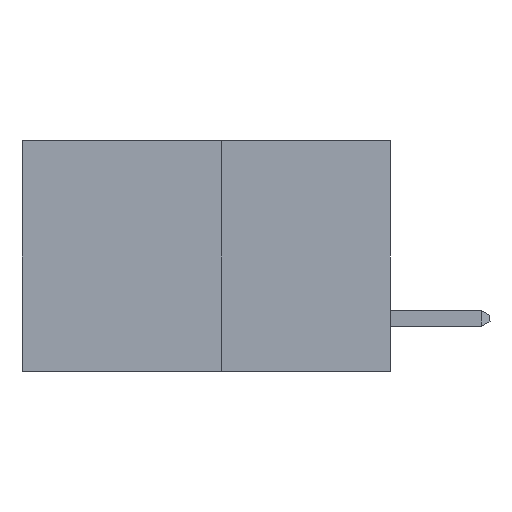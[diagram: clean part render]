
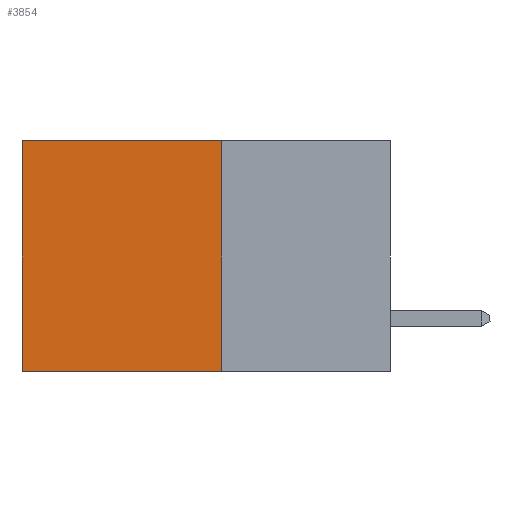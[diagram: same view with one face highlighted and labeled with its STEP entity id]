
A CAD part, left-side view. The second image highlights one B-rep face of the part: STEP entity #3854.
In plain terms, the highlighted planar face has unit normal (-1, 0, 0).
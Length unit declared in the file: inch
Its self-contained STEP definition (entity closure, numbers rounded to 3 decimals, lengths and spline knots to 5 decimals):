
#14 = DIRECTION ( 'NONE',  ( 0., 0., -1. ) ) ;
#146 = ORIENTED_EDGE ( 'NONE', *, *, #3986, .F. ) ;
#190 = CARTESIAN_POINT ( 'NONE',  ( 0.277, 0.59, 0. ) ) ;
#268 = CARTESIAN_POINT ( 'NONE',  ( 0.277, 0.59, -0.37 ) ) ;
#937 = VECTOR ( 'NONE', #4567, 39.37008 ) ;
#1037 = LINE ( 'NONE', #7897, #3661 ) ;
#1048 = EDGE_LOOP ( 'NONE', ( #4002, #146, #6944, #7452 ) ) ;
#1331 = EDGE_CURVE ( 'NONE', #8958, #6787, #9194, .T. ) ;
#1974 = CARTESIAN_POINT ( 'NONE',  ( 0.277, 0.27, -0.37 ) ) ;
#2845 = VECTOR ( 'NONE', #14, 39.37008 ) ;
#3661 = VECTOR ( 'NONE', #10886, 39.37008 ) ;
#3678 = CARTESIAN_POINT ( 'NONE',  ( 0.277, 0.59, -0.37 ) ) ;
#3854 = ADVANCED_FACE ( 'NONE', ( #10508 ), #5303, .F. ) ;
#3986 = EDGE_CURVE ( 'NONE', #6787, #7131, #1037, .T. ) ;
#4002 = ORIENTED_EDGE ( 'NONE', *, *, #5489, .T. ) ;
#4567 = DIRECTION ( 'NONE',  ( 0., 0., -1. ) ) ;
#4999 = AXIS2_PLACEMENT_3D ( 'NONE', #5412, #5261, #5279 ) ;
#5053 = CARTESIAN_POINT ( 'NONE',  ( 0.277, 0.27, 0. ) ) ;
#5261 = DIRECTION ( 'NONE',  ( 1., 0., 0. ) ) ;
#5279 = DIRECTION ( 'NONE',  ( 0., 0., -1. ) ) ;
#5303 = PLANE ( 'NONE',  #4999 ) ;
#5412 = CARTESIAN_POINT ( 'NONE',  ( 0.277, 0.27, -0.37 ) ) ;
#5477 = VERTEX_POINT ( 'NONE', #190 ) ;
#5489 = EDGE_CURVE ( 'NONE', #5477, #7131, #8117, .T. ) ;
#5587 = VECTOR ( 'NONE', #10039, 39.37008 ) ;
#6170 = CARTESIAN_POINT ( 'NONE',  ( 0.277, 0.27, -0.37 ) ) ;
#6787 = VERTEX_POINT ( 'NONE', #6170 ) ;
#6944 = ORIENTED_EDGE ( 'NONE', *, *, #1331, .F. ) ;
#7131 = VERTEX_POINT ( 'NONE', #3678 ) ;
#7452 = ORIENTED_EDGE ( 'NONE', *, *, #10443, .T. ) ;
#7897 = CARTESIAN_POINT ( 'NONE',  ( 0.277, 0.27, -0.37 ) ) ;
#8117 = LINE ( 'NONE', #268, #2845 ) ;
#8958 = VERTEX_POINT ( 'NONE', #9637 ) ;
#9194 = LINE ( 'NONE', #1974, #937 ) ;
#9637 = CARTESIAN_POINT ( 'NONE',  ( 0.277, 0.27, 0. ) ) ;
#10039 = DIRECTION ( 'NONE',  ( 0., 1., 0. ) ) ;
#10443 = EDGE_CURVE ( 'NONE', #8958, #5477, #10845, .T. ) ;
#10508 = FACE_OUTER_BOUND ( 'NONE', #1048, .T. ) ;
#10845 = LINE ( 'NONE', #5053, #5587 ) ;
#10886 = DIRECTION ( 'NONE',  ( 0., 1., 0. ) ) ;
